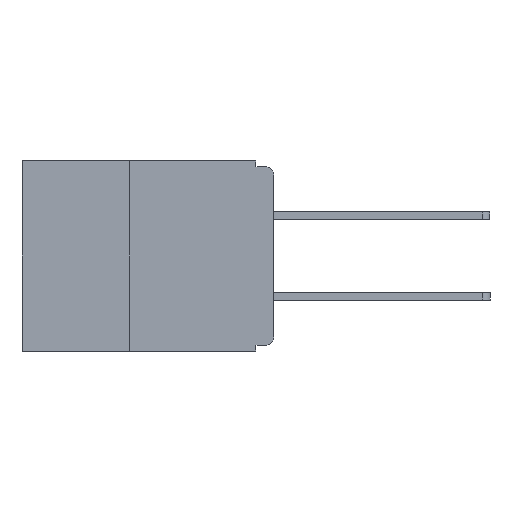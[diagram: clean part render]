
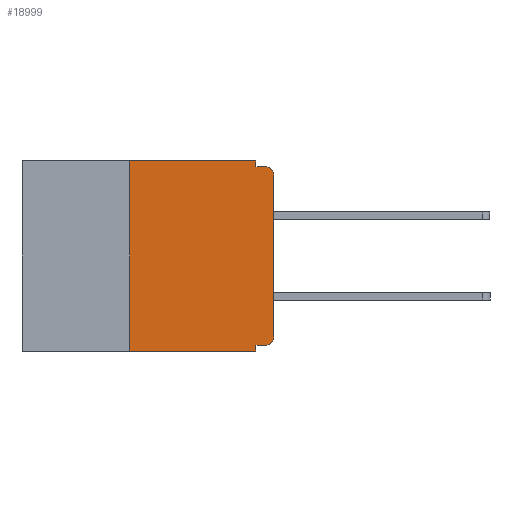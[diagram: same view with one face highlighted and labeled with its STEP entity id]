
A CAD part, left-side view. The second image highlights one B-rep face of the part: STEP entity #18999.
In plain terms, the highlighted planar face has unit normal (-1, 0, 0).
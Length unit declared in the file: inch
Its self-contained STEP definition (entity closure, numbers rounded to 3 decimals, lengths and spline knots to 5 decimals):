
#613 = ORIENTED_EDGE ( 'NONE', *, *, #2829, .T. ) ;
#636 = CARTESIAN_POINT ( 'NONE',  ( 0., 0.031, 0. ) ) ;
#739 = CARTESIAN_POINT ( 'NONE',  ( 0., 0.015, -0.305 ) ) ;
#939 = VERTEX_POINT ( 'NONE', #8682 ) ;
#1220 = VERTEX_POINT ( 'NONE', #7352 ) ;
#2101 = DIRECTION ( 'NONE',  ( 0., 0., -1. ) ) ;
#2182 = EDGE_CURVE ( 'NONE', #16607, #8829, #11706, .T. ) ;
#2282 = VERTEX_POINT ( 'NONE', #30081 ) ;
#2829 = EDGE_CURVE ( 'NONE', #1220, #2282, #7428, .T. ) ;
#4098 = LINE ( 'NONE', #23005, #29133 ) ;
#4283 = CARTESIAN_POINT ( 'NONE',  ( 0., 0.437, 0. ) ) ;
#4469 = LINE ( 'NONE', #23717, #10321 ) ;
#4490 = LINE ( 'NONE', #14831, #10348 ) ;
#5686 = VECTOR ( 'NONE', #23863, 39.37008 ) ;
#6441 = AXIS2_PLACEMENT_3D ( 'NONE', #4283, #9310, #26184 ) ;
#6528 = ORIENTED_EDGE ( 'NONE', *, *, #29855, .F. ) ;
#6783 = PLANE ( 'NONE',  #6441 ) ;
#7028 = CIRCLE ( 'NONE', #8500, 0.015 ) ;
#7352 = CARTESIAN_POINT ( 'NONE',  ( 0., 0.015, -0.32 ) ) ;
#7428 = CIRCLE ( 'NONE', #11673, 0.015 ) ;
#7605 = VERTEX_POINT ( 'NONE', #17748 ) ;
#8093 = ORIENTED_EDGE ( 'NONE', *, *, #25315, .F. ) ;
#8309 = EDGE_LOOP ( 'NONE', ( #25476, #11572, #30344, #8093, #25161, #6528, #29954, #23652, #21346, #613 ) ) ;
#8456 = DIRECTION ( 'NONE',  ( 0., 0., -1. ) ) ;
#8500 = AXIS2_PLACEMENT_3D ( 'NONE', #31116, #16870, #2101 ) ;
#8682 = CARTESIAN_POINT ( 'NONE',  ( 0., 0., -0.025 ) ) ;
#8774 = VERTEX_POINT ( 'NONE', #24898 ) ;
#8829 = VERTEX_POINT ( 'NONE', #636 ) ;
#9310 = DIRECTION ( 'NONE',  ( 1., 0., 0. ) ) ;
#10321 = VECTOR ( 'NONE', #26103, 39.37008 ) ;
#10348 = VECTOR ( 'NONE', #29130, 39.37008 ) ;
#10551 = VECTOR ( 'NONE', #13525, 39.37008 ) ;
#11053 = CARTESIAN_POINT ( 'NONE',  ( 0., 0.031, 0. ) ) ;
#11538 = LINE ( 'NONE', #30882, #5686 ) ;
#11572 = ORIENTED_EDGE ( 'NONE', *, *, #17233, .T. ) ;
#11673 = AXIS2_PLACEMENT_3D ( 'NONE', #739, #25841, #25836 ) ;
#11706 = LINE ( 'NONE', #21654, #23768 ) ;
#11961 = FACE_OUTER_BOUND ( 'NONE', #8309, .T. ) ;
#12301 = DIRECTION ( 'NONE',  ( 0., -1., 0. ) ) ;
#12812 = VERTEX_POINT ( 'NONE', #15818 ) ;
#12983 = EDGE_CURVE ( 'NONE', #8774, #21331, #22215, .T. ) ;
#13525 = DIRECTION ( 'NONE',  ( 0., 0., -1. ) ) ;
#14831 = CARTESIAN_POINT ( 'NONE',  ( 0., 0.25, -0.33 ) ) ;
#15421 = CARTESIAN_POINT ( 'NONE',  ( 0., 0.015, -0.01 ) ) ;
#15818 = CARTESIAN_POINT ( 'NONE',  ( 0., 0.031, -0.01 ) ) ;
#16576 = VECTOR ( 'NONE', #28352, 39.37008 ) ;
#16607 = VERTEX_POINT ( 'NONE', #24046 ) ;
#16870 = DIRECTION ( 'NONE',  ( -1., 0., 0. ) ) ;
#17233 = EDGE_CURVE ( 'NONE', #939, #30673, #7028, .T. ) ;
#17748 = CARTESIAN_POINT ( 'NONE',  ( 0., 0.031, -0.32 ) ) ;
#18999 = ADVANCED_FACE ( 'NONE', ( #11961 ), #6783, .F. ) ;
#19665 = EDGE_CURVE ( 'NONE', #1220, #7605, #11538, .T. ) ;
#20094 = EDGE_CURVE ( 'NONE', #7605, #21331, #4098, .T. ) ;
#20289 = EDGE_CURVE ( 'NONE', #2282, #939, #4469, .T. ) ;
#20900 = EDGE_CURVE ( 'NONE', #12812, #30673, #30549, .T. ) ;
#21331 = VERTEX_POINT ( 'NONE', #28133 ) ;
#21346 = ORIENTED_EDGE ( 'NONE', *, *, #19665, .F. ) ;
#21654 = CARTESIAN_POINT ( 'NONE',  ( 0., 0.437, 0. ) ) ;
#22215 = LINE ( 'NONE', #30691, #16576 ) ;
#23005 = CARTESIAN_POINT ( 'NONE',  ( 0., 0.031, -0.33 ) ) ;
#23652 = ORIENTED_EDGE ( 'NONE', *, *, #20094, .F. ) ;
#23717 = CARTESIAN_POINT ( 'NONE',  ( 0., 0., 0. ) ) ;
#23768 = VECTOR ( 'NONE', #12301, 39.37008 ) ;
#23863 = DIRECTION ( 'NONE',  ( 0., 1., 0. ) ) ;
#24003 = DIRECTION ( 'NONE',  ( 0., -1., 0. ) ) ;
#24046 = CARTESIAN_POINT ( 'NONE',  ( 0., 0.25, 0. ) ) ;
#24898 = CARTESIAN_POINT ( 'NONE',  ( 0., 0.25, -0.33 ) ) ;
#25161 = ORIENTED_EDGE ( 'NONE', *, *, #2182, .F. ) ;
#25315 = EDGE_CURVE ( 'NONE', #8829, #12812, #29706, .T. ) ;
#25476 = ORIENTED_EDGE ( 'NONE', *, *, #20289, .T. ) ;
#25836 = DIRECTION ( 'NONE',  ( 0., 0., -1. ) ) ;
#25841 = DIRECTION ( 'NONE',  ( -1., 0., 0. ) ) ;
#26103 = DIRECTION ( 'NONE',  ( 0., 0., 1. ) ) ;
#26184 = DIRECTION ( 'NONE',  ( 0., 0., -1. ) ) ;
#26385 = CARTESIAN_POINT ( 'NONE',  ( 0., 0., -0.01 ) ) ;
#28133 = CARTESIAN_POINT ( 'NONE',  ( 0., 0.031, -0.33 ) ) ;
#28352 = DIRECTION ( 'NONE',  ( 0., -1., 0. ) ) ;
#29130 = DIRECTION ( 'NONE',  ( 0., 0., 1. ) ) ;
#29133 = VECTOR ( 'NONE', #8456, 39.37008 ) ;
#29706 = LINE ( 'NONE', #11053, #10551 ) ;
#29855 = EDGE_CURVE ( 'NONE', #8774, #16607, #4490, .T. ) ;
#29954 = ORIENTED_EDGE ( 'NONE', *, *, #12983, .T. ) ;
#30081 = CARTESIAN_POINT ( 'NONE',  ( 0., 0., -0.305 ) ) ;
#30344 = ORIENTED_EDGE ( 'NONE', *, *, #20900, .F. ) ;
#30549 = LINE ( 'NONE', #26385, #31270 ) ;
#30673 = VERTEX_POINT ( 'NONE', #15421 ) ;
#30691 = CARTESIAN_POINT ( 'NONE',  ( 0., 0.437, -0.33 ) ) ;
#30882 = CARTESIAN_POINT ( 'NONE',  ( 0., 0., -0.32 ) ) ;
#31116 = CARTESIAN_POINT ( 'NONE',  ( 0., 0.015, -0.025 ) ) ;
#31270 = VECTOR ( 'NONE', #24003, 39.37008 ) ;
